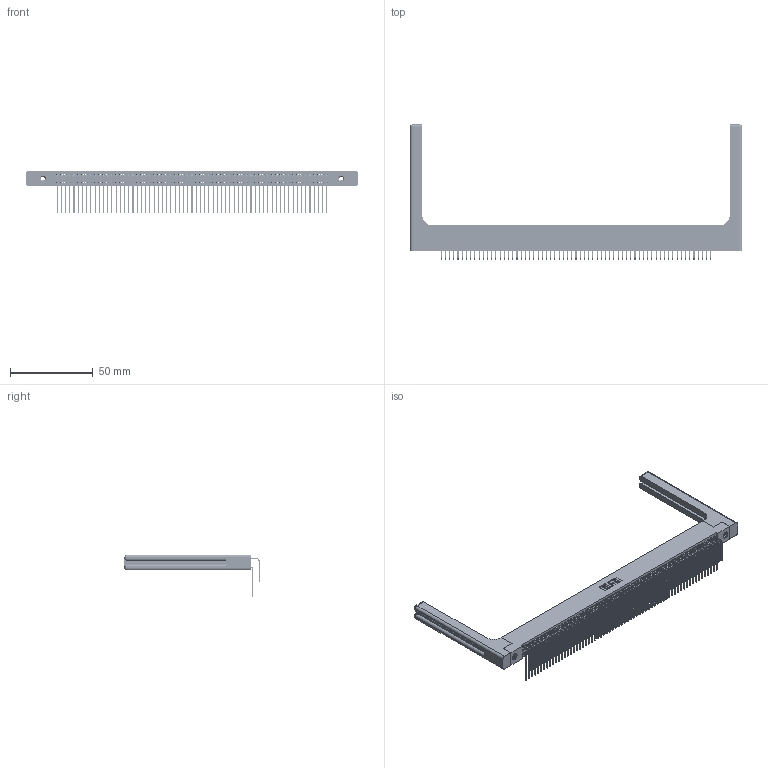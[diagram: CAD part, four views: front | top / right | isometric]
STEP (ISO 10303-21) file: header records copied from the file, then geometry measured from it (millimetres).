
FILE_DESCRIPTION (( 'STEP AP203' ), '1' );
FILE_NAME ('395-130-559-258.STEP', '2019-10-29T00:55:22', ( '' ), ( '' ), 'SwSTEP 2.0', 'SolidWorks 2016', '' );
FILE_SCHEMA (( 'CONFIG_CONTROL_DESIGN' ));
Length unit declared in the file: inch
Products named in the file (6): 345 Part_Flush Mounting Lugs - 0.156 Dia-TH; 345-292-001_558 559 Tail - 1; 345-292-001_559 Tail - 2; 345-250-001_345-250-001-102; 345-220-058_345-220-058; 395-130-559-258
Assembly tree (135 placements, depth 2):
  395-130-559-258
    345 Part_Flush Mounting Lugs - 0.156 Dia-TH
    345-292-001_558 559 Tail - 1  x65
    345-292-001_559 Tail - 2  x65
    345-250-001_345-250-001-102  x2
    345-220-058_345-220-058  x2
Bounding box: 200.13 x 81.52 x 25.53 mm (x, y, z)
Volume: 28879 mm3; surface area: 39191.2 mm2
Topology: 135 solids, 135 shells, 7142 faces, 21157 edges, 13910 vertices
Faces by surface type: plane 4778, cylinder 2304, bspline 36, cone 12, sphere 8, torus 4
Entity records: 54738 total; most frequent: CARTESIAN_POINT 10192, ORIENTED_EDGE 8872, DIRECTION 7864, EDGE_CURVE 4436, VECTOR 3912, LINE 3912, VERTEX_POINT 2946, AXIS2_PLACEMENT_3D 1976
